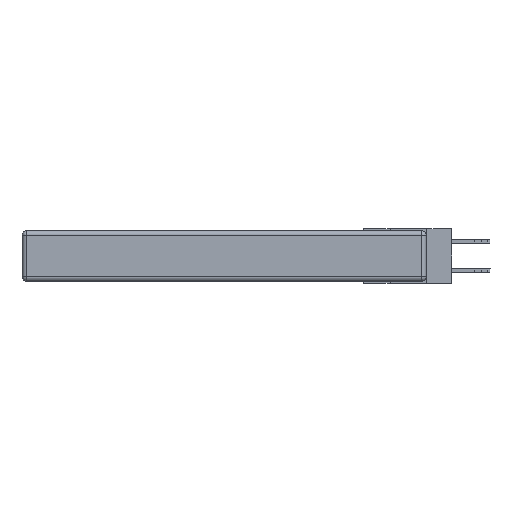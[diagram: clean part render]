
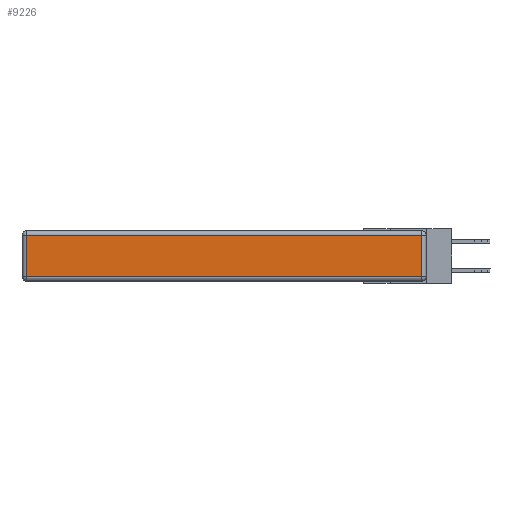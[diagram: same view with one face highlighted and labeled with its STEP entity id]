
A CAD part, left-side view. The second image highlights one B-rep face of the part: STEP entity #9226.
In plain terms, the highlighted planar face has unit normal (-1, 0, 0).
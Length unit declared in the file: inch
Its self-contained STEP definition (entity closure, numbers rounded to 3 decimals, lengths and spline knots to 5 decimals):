
#24 = CARTESIAN_POINT ( 'NONE',  ( 0., 0.03, -0.03 ) ) ;
#341 = CARTESIAN_POINT ( 'NONE',  ( 0., 0.03, -0.343 ) ) ;
#484 = EDGE_CURVE ( 'NONE', #10523, #2842, #5562, .T. ) ;
#585 = ORIENTED_EDGE ( 'NONE', *, *, #484, .T. ) ;
#983 = ORIENTED_EDGE ( 'NONE', *, *, #7443, .T. ) ;
#1103 = CARTESIAN_POINT ( 'NONE',  ( 0., 0.03, -0.313 ) ) ;
#1169 = CARTESIAN_POINT ( 'NONE',  ( 0., 2.75, -0.03 ) ) ;
#1216 = CARTESIAN_POINT ( 'NONE',  ( 0., 2.72, -0.343 ) ) ;
#1381 = DIRECTION ( 'NONE',  ( 0., 0., 1. ) ) ;
#1497 = EDGE_CURVE ( 'NONE', #13217, #3158, #5184, .T. ) ;
#1545 = LINE ( 'NONE', #341, #13289 ) ;
#1745 = ORIENTED_EDGE ( 'NONE', *, *, #3890, .T. ) ;
#2258 = DIRECTION ( 'NONE',  ( 0., 1., 0. ) ) ;
#2842 = VERTEX_POINT ( 'NONE', #11050 ) ;
#3158 = VERTEX_POINT ( 'NONE', #1103 ) ;
#3601 = EDGE_LOOP ( 'NONE', ( #9711, #983, #585, #1745 ) ) ;
#3878 = LINE ( 'NONE', #1216, #4044 ) ;
#3890 = EDGE_CURVE ( 'NONE', #2842, #13217, #3878, .T. ) ;
#4044 = VECTOR ( 'NONE', #8830, 39.37008 ) ;
#4618 = FACE_OUTER_BOUND ( 'NONE', #3601, .T. ) ;
#5184 = LINE ( 'NONE', #7910, #13831 ) ;
#5562 = LINE ( 'NONE', #1169, #7258 ) ;
#5683 = DIRECTION ( 'NONE',  ( 0., 0., 1. ) ) ;
#5781 = PLANE ( 'NONE',  #7851 ) ;
#6830 = DIRECTION ( 'NONE',  ( -1., 0., 0. ) ) ;
#7258 = VECTOR ( 'NONE', #2258, 39.37008 ) ;
#7419 = CARTESIAN_POINT ( 'NONE',  ( 0., 2.72, -0.313 ) ) ;
#7443 = EDGE_CURVE ( 'NONE', #3158, #10523, #1545, .T. ) ;
#7810 = DIRECTION ( 'NONE',  ( 0., -1., 0. ) ) ;
#7851 = AXIS2_PLACEMENT_3D ( 'NONE', #12211, #6830, #5683 ) ;
#7910 = CARTESIAN_POINT ( 'NONE',  ( 0., 0., -0.313 ) ) ;
#8830 = DIRECTION ( 'NONE',  ( 0., 0., -1. ) ) ;
#9226 = ADVANCED_FACE ( 'NONE', ( #4618 ), #5781, .T. ) ;
#9711 = ORIENTED_EDGE ( 'NONE', *, *, #1497, .T. ) ;
#10523 = VERTEX_POINT ( 'NONE', #24 ) ;
#11050 = CARTESIAN_POINT ( 'NONE',  ( 0., 2.72, -0.03 ) ) ;
#12211 = CARTESIAN_POINT ( 'NONE',  ( 0., 0., -0.343 ) ) ;
#13217 = VERTEX_POINT ( 'NONE', #7419 ) ;
#13289 = VECTOR ( 'NONE', #1381, 39.37008 ) ;
#13831 = VECTOR ( 'NONE', #7810, 39.37008 ) ;
